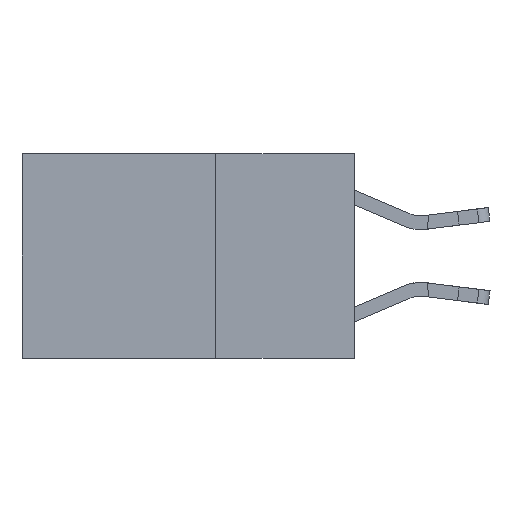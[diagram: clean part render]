
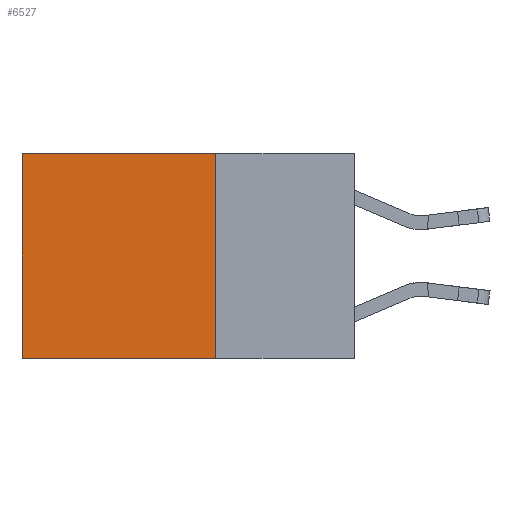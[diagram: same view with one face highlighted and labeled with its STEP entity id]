
A CAD part, left-side view. The second image highlights one B-rep face of the part: STEP entity #6527.
In plain terms, the highlighted planar face has unit normal (-1, 0, 0).
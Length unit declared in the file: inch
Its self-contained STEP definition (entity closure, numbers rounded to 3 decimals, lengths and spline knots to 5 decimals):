
#165 = EDGE_CURVE ( 'NONE', #20172, #5745, #236, .T. ) ;
#236 = LINE ( 'NONE', #20385, #11702 ) ;
#698 = EDGE_CURVE ( 'NONE', #20172, #20255, #5025, .T. ) ;
#854 = CARTESIAN_POINT ( 'NONE',  ( 0.2625, 0.25, -0.37 ) ) ;
#2552 = LINE ( 'NONE', #4179, #12734 ) ;
#3534 = ORIENTED_EDGE ( 'NONE', *, *, #165, .F. ) ;
#4179 = CARTESIAN_POINT ( 'NONE',  ( 0.2625, 0.6, 0. ) ) ;
#5025 = LINE ( 'NONE', #24741, #5676 ) ;
#5676 = VECTOR ( 'NONE', #14712, 39.37008 ) ;
#5745 = VERTEX_POINT ( 'NONE', #854 ) ;
#6527 = ADVANCED_FACE ( 'NONE', ( #16750 ), #7519, .F. ) ;
#6699 = DIRECTION ( 'NONE',  ( 0., 0., -1. ) ) ;
#7115 = ORIENTED_EDGE ( 'NONE', *, *, #22939, .T. ) ;
#7519 = PLANE ( 'NONE',  #11104 ) ;
#7606 = DIRECTION ( 'NONE',  ( 1., 0., 0. ) ) ;
#7794 = DIRECTION ( 'NONE',  ( 0., 1., 0. ) ) ;
#8833 = CARTESIAN_POINT ( 'NONE',  ( 0.2625, 0.6, 0. ) ) ;
#9429 = ORIENTED_EDGE ( 'NONE', *, *, #21757, .F. ) ;
#9619 = VECTOR ( 'NONE', #7794, 39.37008 ) ;
#10260 = EDGE_LOOP ( 'NONE', ( #7115, #9429, #3534, #15780 ) ) ;
#11104 = AXIS2_PLACEMENT_3D ( 'NONE', #19698, #7606, #21726 ) ;
#11702 = VECTOR ( 'NONE', #6699, 39.37008 ) ;
#12734 = VECTOR ( 'NONE', #14250, 39.37008 ) ;
#12809 = VERTEX_POINT ( 'NONE', #13934 ) ;
#13934 = CARTESIAN_POINT ( 'NONE',  ( 0.2625, 0.6, -0.37 ) ) ;
#14250 = DIRECTION ( 'NONE',  ( 0., 0., -1. ) ) ;
#14712 = DIRECTION ( 'NONE',  ( 0., 1., 0. ) ) ;
#14743 = CARTESIAN_POINT ( 'NONE',  ( 0.2625, 0.25, 0. ) ) ;
#15780 = ORIENTED_EDGE ( 'NONE', *, *, #698, .T. ) ;
#16750 = FACE_OUTER_BOUND ( 'NONE', #10260, .T. ) ;
#17862 = CARTESIAN_POINT ( 'NONE',  ( 0.2625, 0.25, -0.37 ) ) ;
#19698 = CARTESIAN_POINT ( 'NONE',  ( 0.2625, 0.25, 0. ) ) ;
#20172 = VERTEX_POINT ( 'NONE', #14743 ) ;
#20255 = VERTEX_POINT ( 'NONE', #8833 ) ;
#20385 = CARTESIAN_POINT ( 'NONE',  ( 0.2625, 0.25, 0. ) ) ;
#21726 = DIRECTION ( 'NONE',  ( 0., 0., -1. ) ) ;
#21757 = EDGE_CURVE ( 'NONE', #5745, #12809, #24442, .T. ) ;
#22939 = EDGE_CURVE ( 'NONE', #20255, #12809, #2552, .T. ) ;
#24442 = LINE ( 'NONE', #17862, #9619 ) ;
#24741 = CARTESIAN_POINT ( 'NONE',  ( 0.2625, 0.25, 0. ) ) ;
